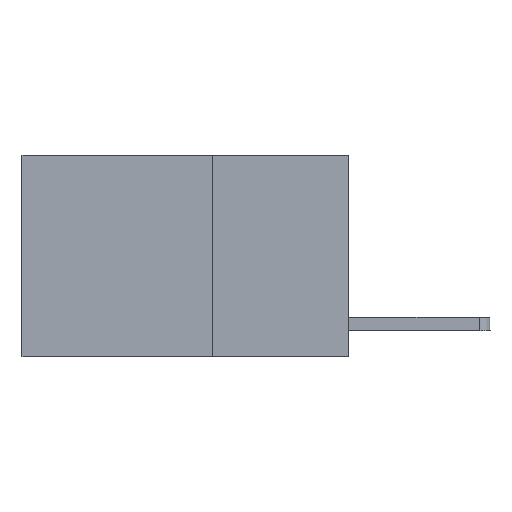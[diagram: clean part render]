
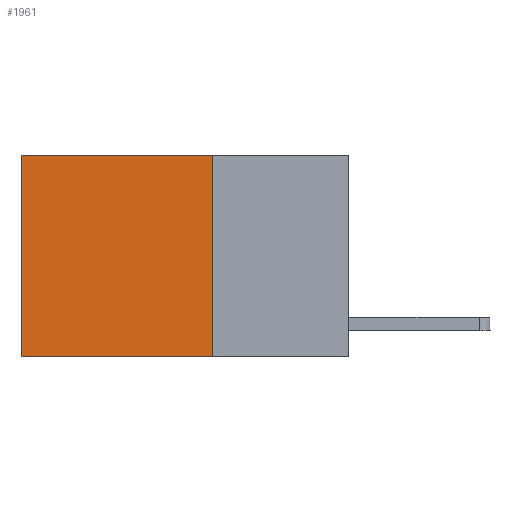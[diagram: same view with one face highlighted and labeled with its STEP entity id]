
A CAD part, left-side view. The second image highlights one B-rep face of the part: STEP entity #1961.
In plain terms, the highlighted planar face has unit normal (-1, 0, 0).
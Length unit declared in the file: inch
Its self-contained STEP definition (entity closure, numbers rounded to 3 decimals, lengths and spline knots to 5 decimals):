
#33 = ORIENTED_EDGE ( 'NONE', *, *, #1761, .T. ) ;
#195 = LINE ( 'NONE', #994, #400 ) ;
#400 = VECTOR ( 'NONE', #5861, 39.37008 ) ;
#565 = FACE_OUTER_BOUND ( 'NONE', #2754, .T. ) ;
#651 = PLANE ( 'NONE',  #5936 ) ;
#864 = CARTESIAN_POINT ( 'NONE',  ( 0.2625, 0.25, 0. ) ) ;
#994 = CARTESIAN_POINT ( 'NONE',  ( 0.2625, 0.6, 0. ) ) ;
#1079 = ORIENTED_EDGE ( 'NONE', *, *, #6673, .T. ) ;
#1114 = EDGE_CURVE ( 'NONE', #5024, #7560, #9212, .T. ) ;
#1334 = CARTESIAN_POINT ( 'NONE',  ( 0.2625, 0.25, 0. ) ) ;
#1499 = CARTESIAN_POINT ( 'NONE',  ( 0.2625, 0.25, -0.37 ) ) ;
#1586 = VERTEX_POINT ( 'NONE', #7806 ) ;
#1761 = EDGE_CURVE ( 'NONE', #5024, #1586, #3707, .T. ) ;
#1763 = CARTESIAN_POINT ( 'NONE',  ( 0.2625, 0.6, -0.37 ) ) ;
#1961 = ADVANCED_FACE ( 'NONE', ( #565 ), #651, .F. ) ;
#2016 = DIRECTION ( 'NONE',  ( 1., 0., 0. ) ) ;
#2754 = EDGE_LOOP ( 'NONE', ( #1079, #5401, #5264, #33 ) ) ;
#3042 = DIRECTION ( 'NONE',  ( 0., 1., 0. ) ) ;
#3511 = CARTESIAN_POINT ( 'NONE',  ( 0.2625, 0.25, 0. ) ) ;
#3707 = LINE ( 'NONE', #5760, #4588 ) ;
#3806 = VECTOR ( 'NONE', #7257, 39.37008 ) ;
#4588 = VECTOR ( 'NONE', #3042, 39.37008 ) ;
#4975 = VERTEX_POINT ( 'NONE', #1763 ) ;
#5024 = VERTEX_POINT ( 'NONE', #864 ) ;
#5264 = ORIENTED_EDGE ( 'NONE', *, *, #1114, .F. ) ;
#5401 = ORIENTED_EDGE ( 'NONE', *, *, #5434, .F. ) ;
#5434 = EDGE_CURVE ( 'NONE', #7560, #4975, #8080, .T. ) ;
#5760 = CARTESIAN_POINT ( 'NONE',  ( 0.2625, 0.25, 0. ) ) ;
#5861 = DIRECTION ( 'NONE',  ( 0., 0., -1. ) ) ;
#5936 = AXIS2_PLACEMENT_3D ( 'NONE', #3511, #2016, #7757 ) ;
#5950 = VECTOR ( 'NONE', #8417, 39.37008 ) ;
#6673 = EDGE_CURVE ( 'NONE', #1586, #4975, #195, .T. ) ;
#7257 = DIRECTION ( 'NONE',  ( 0., 1., 0. ) ) ;
#7560 = VERTEX_POINT ( 'NONE', #1499 ) ;
#7757 = DIRECTION ( 'NONE',  ( 0., 0., -1. ) ) ;
#7806 = CARTESIAN_POINT ( 'NONE',  ( 0.2625, 0.6, 0. ) ) ;
#8041 = CARTESIAN_POINT ( 'NONE',  ( 0.2625, 0.25, -0.37 ) ) ;
#8080 = LINE ( 'NONE', #8041, #3806 ) ;
#8417 = DIRECTION ( 'NONE',  ( 0., 0., -1. ) ) ;
#9212 = LINE ( 'NONE', #1334, #5950 ) ;
